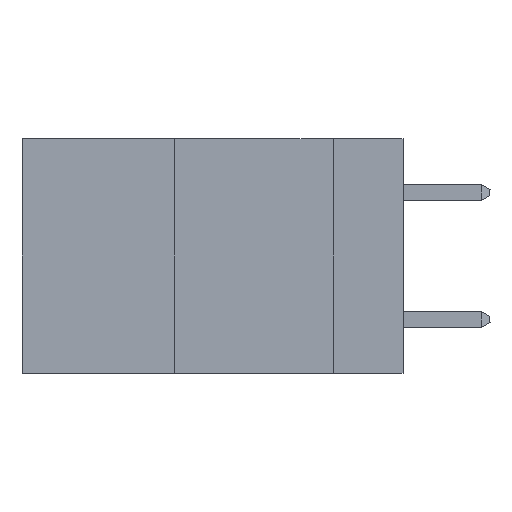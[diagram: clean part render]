
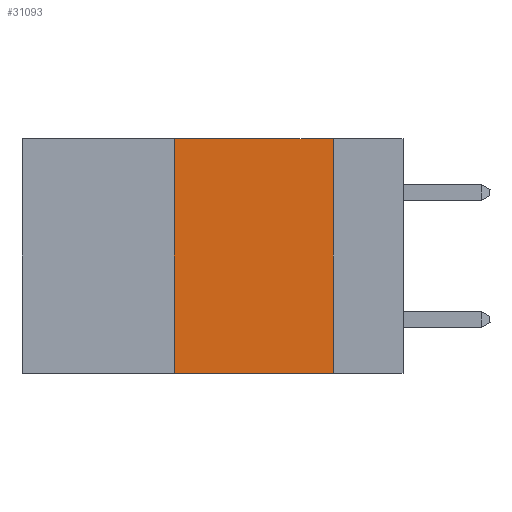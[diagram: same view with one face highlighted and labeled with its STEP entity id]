
A CAD part, left-side view. The second image highlights one B-rep face of the part: STEP entity #31093.
In plain terms, the highlighted planar face has unit normal (-1, 0, 0).
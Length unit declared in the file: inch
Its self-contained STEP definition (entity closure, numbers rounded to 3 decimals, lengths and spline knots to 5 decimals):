
#301 = VERTEX_POINT ( 'NONE', #19149 ) ;
#1492 = DIRECTION ( 'NONE',  ( 0., 0., 1. ) ) ;
#2797 = ORIENTED_EDGE ( 'NONE', *, *, #31029, .F. ) ;
#3386 = VERTEX_POINT ( 'NONE', #19227 ) ;
#4752 = CARTESIAN_POINT ( 'NONE',  ( 0., 0.36, -0.37 ) ) ;
#4883 = VECTOR ( 'NONE', #1492, 39.37008 ) ;
#5000 = LINE ( 'NONE', #13239, #17398 ) ;
#5267 = VERTEX_POINT ( 'NONE', #4752 ) ;
#7782 = DIRECTION ( 'NONE',  ( 1., 0., 0. ) ) ;
#13049 = LINE ( 'NONE', #21193, #18813 ) ;
#13239 = CARTESIAN_POINT ( 'NONE',  ( 0., 0.6, -0.37 ) ) ;
#13659 = CARTESIAN_POINT ( 'NONE',  ( 0., 0.36, 0. ) ) ;
#15740 = DIRECTION ( 'NONE',  ( 0., -1., 0. ) ) ;
#16029 = ORIENTED_EDGE ( 'NONE', *, *, #19072, .F. ) ;
#16443 = DIRECTION ( 'NONE',  ( 0., 0., -1. ) ) ;
#17398 = VECTOR ( 'NONE', #15740, 39.37008 ) ;
#17608 = VERTEX_POINT ( 'NONE', #13659 ) ;
#18032 = LINE ( 'NONE', #30836, #4883 ) ;
#18813 = VECTOR ( 'NONE', #16443, 39.37008 ) ;
#19072 = EDGE_CURVE ( 'NONE', #5267, #17608, #18032, .T. ) ;
#19149 = CARTESIAN_POINT ( 'NONE',  ( 0., 0.11, 0. ) ) ;
#19227 = CARTESIAN_POINT ( 'NONE',  ( 0., 0.11, -0.37 ) ) ;
#19776 = CARTESIAN_POINT ( 'NONE',  ( 0., 0.6, 0. ) ) ;
#20278 = FACE_OUTER_BOUND ( 'NONE', #24066, .T. ) ;
#21193 = CARTESIAN_POINT ( 'NONE',  ( 0., 0.11, 0. ) ) ;
#21799 = VECTOR ( 'NONE', #24651, 39.37008 ) ;
#22526 = PLANE ( 'NONE',  #26831 ) ;
#23923 = EDGE_CURVE ( 'NONE', #301, #3386, #13049, .T. ) ;
#24066 = EDGE_LOOP ( 'NONE', ( #28097, #2797, #16029, #30375 ) ) ;
#24651 = DIRECTION ( 'NONE',  ( 0., -1., 0. ) ) ;
#24950 = DIRECTION ( 'NONE',  ( 0., 0., -1. ) ) ;
#26831 = AXIS2_PLACEMENT_3D ( 'NONE', #29692, #7782, #24950 ) ;
#28097 = ORIENTED_EDGE ( 'NONE', *, *, #23923, .F. ) ;
#28195 = LINE ( 'NONE', #19776, #21799 ) ;
#28339 = EDGE_CURVE ( 'NONE', #5267, #3386, #5000, .T. ) ;
#29692 = CARTESIAN_POINT ( 'NONE',  ( 0., 0.6, 0. ) ) ;
#30375 = ORIENTED_EDGE ( 'NONE', *, *, #28339, .T. ) ;
#30836 = CARTESIAN_POINT ( 'NONE',  ( 0., 0.36, 0. ) ) ;
#31029 = EDGE_CURVE ( 'NONE', #17608, #301, #28195, .T. ) ;
#31093 = ADVANCED_FACE ( 'NONE', ( #20278 ), #22526, .F. ) ;
